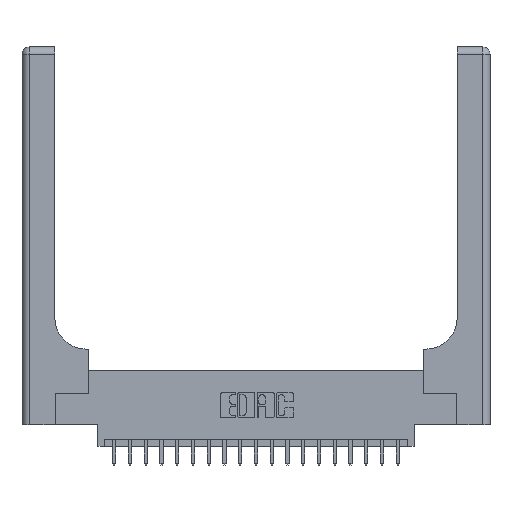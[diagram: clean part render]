
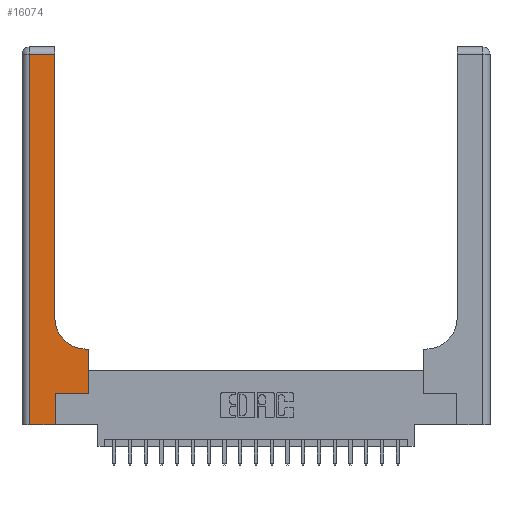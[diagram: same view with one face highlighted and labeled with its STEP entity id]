
A CAD part, top view. The second image highlights one B-rep face of the part: STEP entity #16074.
In plain terms, the highlighted planar face has unit normal (0, 0, 1).
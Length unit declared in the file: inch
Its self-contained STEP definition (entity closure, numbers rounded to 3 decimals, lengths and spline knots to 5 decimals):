
#176 = CARTESIAN_POINT ( 'NONE',  ( 0., 3., 0.37 ) ) ;
#367 = CARTESIAN_POINT ( 'NONE',  ( 0.26, 0.6, 0.37 ) ) ;
#608 = ORIENTED_EDGE ( 'NONE', *, *, #2238, .T. ) ;
#629 = CARTESIAN_POINT ( 'NONE',  ( 0.26, 2.94, 0.37 ) ) ;
#773 = ORIENTED_EDGE ( 'NONE', *, *, #1692, .T. ) ;
#1055 = VERTEX_POINT ( 'NONE', #18578 ) ;
#1692 = EDGE_CURVE ( 'NONE', #3790, #2288, #15142, .T. ) ;
#1699 = ORIENTED_EDGE ( 'NONE', *, *, #8914, .T. ) ;
#1946 = VECTOR ( 'NONE', #19023, 39.37008 ) ;
#2127 = LINE ( 'NONE', #5795, #1946 ) ;
#2180 = LINE ( 'NONE', #7028, #12006 ) ;
#2238 = EDGE_CURVE ( 'NONE', #20841, #14117, #12834, .T. ) ;
#2288 = VERTEX_POINT ( 'NONE', #10787 ) ;
#2495 = CARTESIAN_POINT ( 'NONE',  ( 0.528, 0.25, 0.37 ) ) ;
#2660 = DIRECTION ( 'NONE',  ( 0., 1., 0. ) ) ;
#3277 = EDGE_CURVE ( 'NONE', #1055, #13461, #2180, .T. ) ;
#3440 = VERTEX_POINT ( 'NONE', #19389 ) ;
#3790 = VERTEX_POINT ( 'NONE', #7005 ) ;
#4505 = ORIENTED_EDGE ( 'NONE', *, *, #17983, .T. ) ;
#4686 = LINE ( 'NONE', #19342, #11284 ) ;
#5232 = FACE_OUTER_BOUND ( 'NONE', #5829, .T. ) ;
#5276 = DIRECTION ( 'NONE',  ( 0., -1., 0. ) ) ;
#5349 = PLANE ( 'NONE',  #17829 ) ;
#5795 = CARTESIAN_POINT ( 'NONE',  ( 0., 2.94, 0.37 ) ) ;
#5829 = EDGE_LOOP ( 'NONE', ( #4505, #1699, #14039, #15188, #9757, #608, #18296, #773, #20038 ) ) ;
#6867 = DIRECTION ( 'NONE',  ( 0., 0., -1. ) ) ;
#7005 = CARTESIAN_POINT ( 'NONE',  ( 0.528, 0.6, 0.37 ) ) ;
#7028 = CARTESIAN_POINT ( 'NONE',  ( 0., 0., 0.37 ) ) ;
#7971 = EDGE_CURVE ( 'NONE', #14117, #3790, #12525, .T. ) ;
#8198 = CIRCLE ( 'NONE', #15092, 0.25 ) ;
#8430 = VECTOR ( 'NONE', #19951, 39.37008 ) ;
#8914 = EDGE_CURVE ( 'NONE', #17383, #3440, #2127, .T. ) ;
#9143 = VECTOR ( 'NONE', #5276, 39.37008 ) ;
#9702 = VECTOR ( 'NONE', #19172, 39.37008 ) ;
#9757 = ORIENTED_EDGE ( 'NONE', *, *, #17893, .T. ) ;
#10445 = CARTESIAN_POINT ( 'NONE',  ( 0.528, 0.25, 0.37 ) ) ;
#10537 = VECTOR ( 'NONE', #14340, 39.37008 ) ;
#10787 = CARTESIAN_POINT ( 'NONE',  ( 0.51, 0.6, 0.37 ) ) ;
#10947 = VECTOR ( 'NONE', #12785, 39.37008 ) ;
#11284 = VECTOR ( 'NONE', #2660, 39.37008 ) ;
#12006 = VECTOR ( 'NONE', #15333, 39.37008 ) ;
#12525 = LINE ( 'NONE', #2495, #9702 ) ;
#12785 = DIRECTION ( 'NONE',  ( 0., 1., 0. ) ) ;
#12834 = LINE ( 'NONE', #17459, #10537 ) ;
#13420 = VERTEX_POINT ( 'NONE', #14421 ) ;
#13441 = DIRECTION ( 'NONE',  ( -1., 0., 0. ) ) ;
#13461 = VERTEX_POINT ( 'NONE', #17543 ) ;
#13675 = CARTESIAN_POINT ( 'NONE',  ( 0.51, 0.85, 0.37 ) ) ;
#14016 = EDGE_CURVE ( 'NONE', #3440, #1055, #20043, .T. ) ;
#14039 = ORIENTED_EDGE ( 'NONE', *, *, #14016, .T. ) ;
#14117 = VERTEX_POINT ( 'NONE', #10445 ) ;
#14340 = DIRECTION ( 'NONE',  ( 1., 0., 0. ) ) ;
#14421 = CARTESIAN_POINT ( 'NONE',  ( 0.26, 0.85, 0.37 ) ) ;
#14593 = CARTESIAN_POINT ( 'NONE',  ( 0.265, 0.25, 0.37 ) ) ;
#15092 = AXIS2_PLACEMENT_3D ( 'NONE', #13675, #18610, #20443 ) ;
#15142 = LINE ( 'NONE', #367, #8430 ) ;
#15188 = ORIENTED_EDGE ( 'NONE', *, *, #3277, .T. ) ;
#15333 = DIRECTION ( 'NONE',  ( 1., 0., 0. ) ) ;
#15834 = CARTESIAN_POINT ( 'NONE',  ( 0.265, 0., 0.37 ) ) ;
#16074 = ADVANCED_FACE ( 'NONE', ( #5232 ), #5349, .F. ) ;
#17383 = VERTEX_POINT ( 'NONE', #629 ) ;
#17459 = CARTESIAN_POINT ( 'NONE',  ( 0.265, 0.25, 0.37 ) ) ;
#17543 = CARTESIAN_POINT ( 'NONE',  ( 0.265, 0., 0.37 ) ) ;
#17829 = AXIS2_PLACEMENT_3D ( 'NONE', #176, #6867, #13441 ) ;
#17893 = EDGE_CURVE ( 'NONE', #13461, #20841, #21073, .T. ) ;
#17983 = EDGE_CURVE ( 'NONE', #13420, #17383, #4686, .T. ) ;
#18296 = ORIENTED_EDGE ( 'NONE', *, *, #7971, .T. ) ;
#18529 = EDGE_CURVE ( 'NONE', #2288, #13420, #8198, .T. ) ;
#18578 = CARTESIAN_POINT ( 'NONE',  ( 0.06, 0., 0.37 ) ) ;
#18610 = DIRECTION ( 'NONE',  ( 0., 0., -1. ) ) ;
#19023 = DIRECTION ( 'NONE',  ( -1., 0., 0. ) ) ;
#19172 = DIRECTION ( 'NONE',  ( 0., 1., 0. ) ) ;
#19342 = CARTESIAN_POINT ( 'NONE',  ( 0.26, 3., 0.37 ) ) ;
#19389 = CARTESIAN_POINT ( 'NONE',  ( 0.06, 2.94, 0.37 ) ) ;
#19714 = CARTESIAN_POINT ( 'NONE',  ( 0.06, 3., 0.37 ) ) ;
#19951 = DIRECTION ( 'NONE',  ( -1., 0., 0. ) ) ;
#20038 = ORIENTED_EDGE ( 'NONE', *, *, #18529, .T. ) ;
#20043 = LINE ( 'NONE', #19714, #9143 ) ;
#20443 = DIRECTION ( 'NONE',  ( 1., 0., 0. ) ) ;
#20841 = VERTEX_POINT ( 'NONE', #14593 ) ;
#21073 = LINE ( 'NONE', #15834, #10947 ) ;
